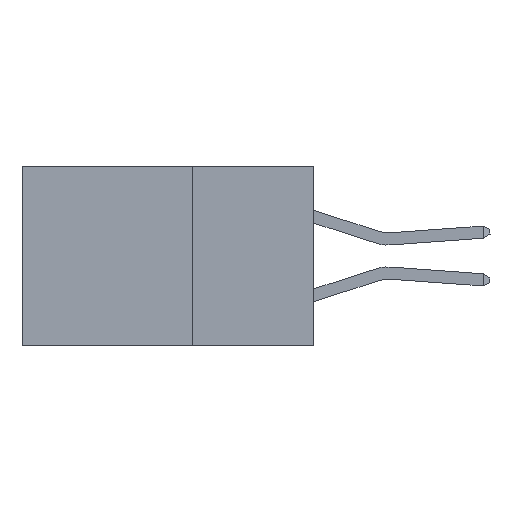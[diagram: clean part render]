
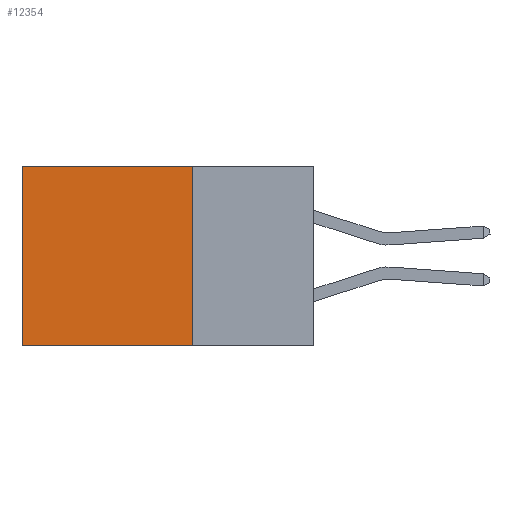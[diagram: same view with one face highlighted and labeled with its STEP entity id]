
A CAD part, left-side view. The second image highlights one B-rep face of the part: STEP entity #12354.
In plain terms, the highlighted planar face has unit normal (-1, 0, 0).
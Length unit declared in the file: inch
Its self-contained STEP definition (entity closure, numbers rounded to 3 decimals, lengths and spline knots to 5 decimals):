
#1025 = CARTESIAN_POINT ( 'NONE',  ( 0.2875, 0.6, 0. ) ) ;
#1034 = VECTOR ( 'NONE', #19301, 39.37008 ) ;
#1076 = DIRECTION ( 'NONE',  ( 0., 0., -1. ) ) ;
#1313 = DIRECTION ( 'NONE',  ( 0., 0., -1. ) ) ;
#1796 = LINE ( 'NONE', #14287, #1034 ) ;
#2398 = EDGE_CURVE ( 'NONE', #10647, #15773, #13552, .T. ) ;
#3118 = CARTESIAN_POINT ( 'NONE',  ( 0.2875, 0.25, -0.37 ) ) ;
#3333 = CARTESIAN_POINT ( 'NONE',  ( 0.2875, 0.6, -0.37 ) ) ;
#3831 = VECTOR ( 'NONE', #4242, 39.37008 ) ;
#4242 = DIRECTION ( 'NONE',  ( 0., 1., 0. ) ) ;
#4327 = CARTESIAN_POINT ( 'NONE',  ( 0.2875, 0.6, 0. ) ) ;
#6277 = VERTEX_POINT ( 'NONE', #19689 ) ;
#6303 = ORIENTED_EDGE ( 'NONE', *, *, #19629, .F. ) ;
#6574 = ORIENTED_EDGE ( 'NONE', *, *, #17373, .T. ) ;
#7209 = CARTESIAN_POINT ( 'NONE',  ( 0.2875, 0.25, 0. ) ) ;
#7839 = ORIENTED_EDGE ( 'NONE', *, *, #15102, .T. ) ;
#8150 = VECTOR ( 'NONE', #1076, 39.37008 ) ;
#8648 = LINE ( 'NONE', #7209, #8150 ) ;
#10109 = AXIS2_PLACEMENT_3D ( 'NONE', #12480, #20371, #1313 ) ;
#10353 = CARTESIAN_POINT ( 'NONE',  ( 0.2875, 0.25, -0.37 ) ) ;
#10647 = VERTEX_POINT ( 'NONE', #3118 ) ;
#10743 = PLANE ( 'NONE',  #10109 ) ;
#10860 = LINE ( 'NONE', #1025, #13634 ) ;
#11987 = DIRECTION ( 'NONE',  ( 0., 0., -1. ) ) ;
#12354 = ADVANCED_FACE ( 'NONE', ( #20286 ), #10743, .F. ) ;
#12407 = ORIENTED_EDGE ( 'NONE', *, *, #2398, .F. ) ;
#12480 = CARTESIAN_POINT ( 'NONE',  ( 0.2875, 0.25, 0. ) ) ;
#13552 = LINE ( 'NONE', #10353, #3831 ) ;
#13634 = VECTOR ( 'NONE', #11987, 39.37008 ) ;
#14287 = CARTESIAN_POINT ( 'NONE',  ( 0.2875, 0.25, 0. ) ) ;
#15102 = EDGE_CURVE ( 'NONE', #6277, #18130, #1796, .T. ) ;
#15773 = VERTEX_POINT ( 'NONE', #3333 ) ;
#17205 = EDGE_LOOP ( 'NONE', ( #6574, #12407, #6303, #7839 ) ) ;
#17373 = EDGE_CURVE ( 'NONE', #18130, #15773, #10860, .T. ) ;
#18130 = VERTEX_POINT ( 'NONE', #4327 ) ;
#19301 = DIRECTION ( 'NONE',  ( 0., 1., 0. ) ) ;
#19629 = EDGE_CURVE ( 'NONE', #6277, #10647, #8648, .T. ) ;
#19689 = CARTESIAN_POINT ( 'NONE',  ( 0.2875, 0.25, 0. ) ) ;
#20286 = FACE_OUTER_BOUND ( 'NONE', #17205, .T. ) ;
#20371 = DIRECTION ( 'NONE',  ( 1., 0., 0. ) ) ;
